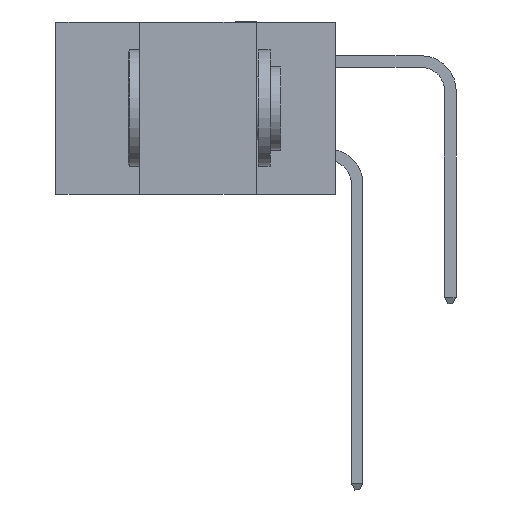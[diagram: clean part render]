
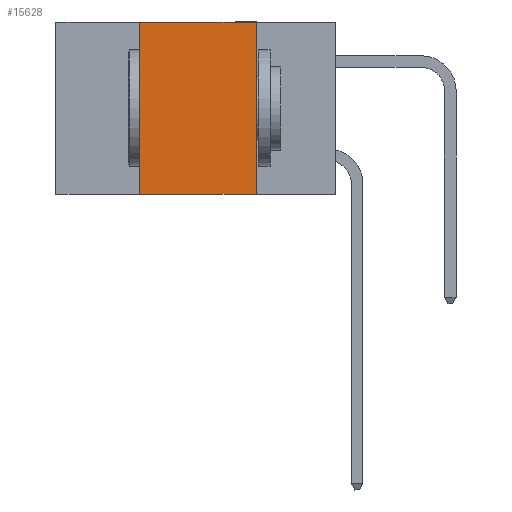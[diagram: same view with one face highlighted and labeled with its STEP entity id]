
A CAD part, left-side view. The second image highlights one B-rep face of the part: STEP entity #15628.
In plain terms, the highlighted planar face has unit normal (-1, 0, 0).
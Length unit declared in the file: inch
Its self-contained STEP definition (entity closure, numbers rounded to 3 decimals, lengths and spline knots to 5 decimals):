
#74 = DIRECTION ( 'NONE',  ( 0., -1., 0. ) ) ;
#909 = VERTEX_POINT ( 'NONE', #17782 ) ;
#932 = CARTESIAN_POINT ( 'NONE',  ( 0., 0.6, -0.37 ) ) ;
#1934 = LINE ( 'NONE', #13201, #9743 ) ;
#2444 = EDGE_CURVE ( 'NONE', #8120, #6475, #2689, .T. ) ;
#2686 = EDGE_CURVE ( 'NONE', #12123, #909, #2931, .T. ) ;
#2689 = LINE ( 'NONE', #932, #14354 ) ;
#2931 = LINE ( 'NONE', #17506, #14564 ) ;
#6475 = VERTEX_POINT ( 'NONE', #17564 ) ;
#6669 = EDGE_LOOP ( 'NONE', ( #11262, #12612, #11501, #18028 ) ) ;
#8120 = VERTEX_POINT ( 'NONE', #11223 ) ;
#9342 = PLANE ( 'NONE',  #9596 ) ;
#9596 = AXIS2_PLACEMENT_3D ( 'NONE', #15166, #19685, #10800 ) ;
#9743 = VECTOR ( 'NONE', #12038, 39.37008 ) ;
#10716 = DIRECTION ( 'NONE',  ( 0., 0., 1. ) ) ;
#10800 = DIRECTION ( 'NONE',  ( 0., 0., -1. ) ) ;
#11223 = CARTESIAN_POINT ( 'NONE',  ( 0., 0.42, -0.37 ) ) ;
#11262 = ORIENTED_EDGE ( 'NONE', *, *, #15921, .F. ) ;
#11367 = FACE_OUTER_BOUND ( 'NONE', #6669, .T. ) ;
#11428 = VECTOR ( 'NONE', #10716, 39.37008 ) ;
#11501 = ORIENTED_EDGE ( 'NONE', *, *, #14315, .F. ) ;
#12038 = DIRECTION ( 'NONE',  ( 0., 0., -1. ) ) ;
#12123 = VERTEX_POINT ( 'NONE', #19315 ) ;
#12612 = ORIENTED_EDGE ( 'NONE', *, *, #2686, .F. ) ;
#13201 = CARTESIAN_POINT ( 'NONE',  ( 0., 0.17, 0. ) ) ;
#13387 = CARTESIAN_POINT ( 'NONE',  ( 0., 0.42, 0. ) ) ;
#14315 = EDGE_CURVE ( 'NONE', #8120, #12123, #18841, .T. ) ;
#14354 = VECTOR ( 'NONE', #74, 39.37008 ) ;
#14564 = VECTOR ( 'NONE', #16243, 39.37008 ) ;
#15166 = CARTESIAN_POINT ( 'NONE',  ( 0., 0.6, 0. ) ) ;
#15628 = ADVANCED_FACE ( 'NONE', ( #11367 ), #9342, .F. ) ;
#15921 = EDGE_CURVE ( 'NONE', #909, #6475, #1934, .T. ) ;
#16243 = DIRECTION ( 'NONE',  ( 0., -1., 0. ) ) ;
#17506 = CARTESIAN_POINT ( 'NONE',  ( 0., 0.6, 0. ) ) ;
#17564 = CARTESIAN_POINT ( 'NONE',  ( 0., 0.17, -0.37 ) ) ;
#17782 = CARTESIAN_POINT ( 'NONE',  ( 0., 0.17, 0. ) ) ;
#18028 = ORIENTED_EDGE ( 'NONE', *, *, #2444, .T. ) ;
#18841 = LINE ( 'NONE', #13387, #11428 ) ;
#19315 = CARTESIAN_POINT ( 'NONE',  ( 0., 0.42, 0. ) ) ;
#19685 = DIRECTION ( 'NONE',  ( 1., 0., 0. ) ) ;
